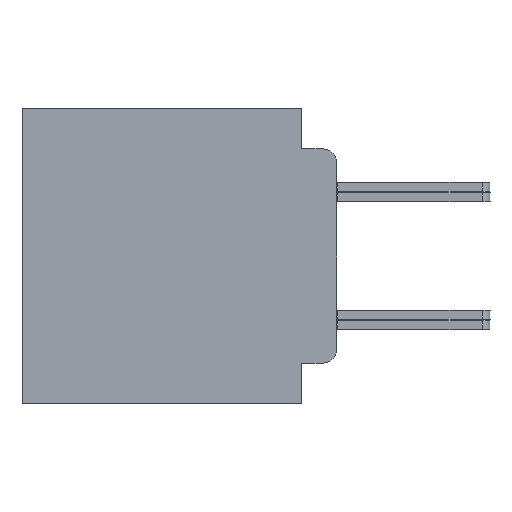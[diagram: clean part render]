
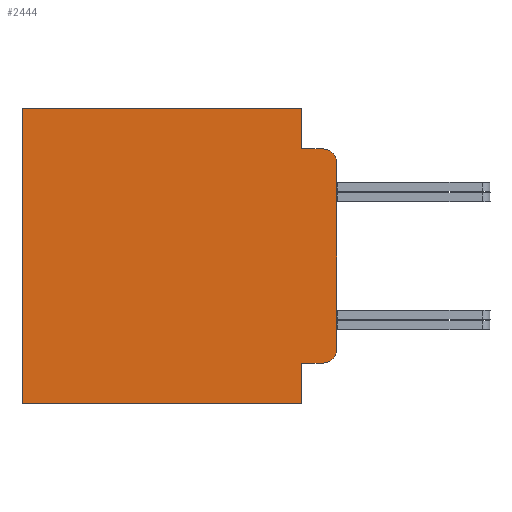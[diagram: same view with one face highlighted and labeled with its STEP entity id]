
A CAD part, left-side view. The second image highlights one B-rep face of the part: STEP entity #2444.
In plain terms, the highlighted planar face has unit normal (-1, 0, 0).
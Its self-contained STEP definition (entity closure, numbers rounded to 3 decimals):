
#29 = VERTEX_POINT ( 'NONE', #157 ) ;
#91 = EDGE_CURVE ( 'NONE', #19798, #8609, #27582, .T. ) ;
#157 = CARTESIAN_POINT ( 'NONE',  ( -67.462, 0., -3.467 ) ) ;
#174 = CARTESIAN_POINT ( 'NONE',  ( -67.462, 1.295, -3.975 ) ) ;
#429 = ORIENTED_EDGE ( 'NONE', *, *, #22593, .F. ) ;
#499 = VERTEX_POINT ( 'NONE', #3277 ) ;
#1486 = VERTEX_POINT ( 'NONE', #13337 ) ;
#2215 = CARTESIAN_POINT ( 'NONE',  ( -67.462, 0.508, 3.467 ) ) ;
#2444 = ADVANCED_FACE ( 'NONE', ( #26117 ), #5662, .F. ) ;
#3277 = CARTESIAN_POINT ( 'NONE',  ( -67.462, 0.508, -3.975 ) ) ;
#3463 = CARTESIAN_POINT ( 'NONE',  ( -67.462, 0., -5.486 ) ) ;
#3476 = CARTESIAN_POINT ( 'NONE',  ( -67.462, 1.295, 0. ) ) ;
#3770 = CARTESIAN_POINT ( 'NONE',  ( -67.462, 1.295, 0. ) ) ;
#4053 = DIRECTION ( 'NONE',  ( 0., 0., -1. ) ) ;
#4057 = LINE ( 'NONE', #3476, #26581 ) ;
#4779 = CARTESIAN_POINT ( 'NONE',  ( -67.462, 1.295, -5.486 ) ) ;
#5070 = LINE ( 'NONE', #24773, #21764 ) ;
#5470 = DIRECTION ( 'NONE',  ( 0., 0., -1. ) ) ;
#5475 = LINE ( 'NONE', #3463, #10943 ) ;
#5662 = PLANE ( 'NONE',  #19592 ) ;
#5704 = LINE ( 'NONE', #23634, #21716 ) ;
#5741 = VECTOR ( 'NONE', #18040, 1000. ) ;
#5996 = EDGE_CURVE ( 'NONE', #14584, #23016, #4057, .T. ) ;
#7024 = EDGE_CURVE ( 'NONE', #23016, #8609, #5070, .T. ) ;
#7458 = CARTESIAN_POINT ( 'NONE',  ( -67.462, 11.684, 5.486 ) ) ;
#8059 = CARTESIAN_POINT ( 'NONE',  ( -67.462, 0., -5.486 ) ) ;
#8399 = EDGE_CURVE ( 'NONE', #19581, #1486, #12910, .T. ) ;
#8609 = VERTEX_POINT ( 'NONE', #19529 ) ;
#8669 = ORIENTED_EDGE ( 'NONE', *, *, #8399, .F. ) ;
#8825 = VECTOR ( 'NONE', #16134, 1000. ) ;
#8961 = VERTEX_POINT ( 'NONE', #10941 ) ;
#9251 = ORIENTED_EDGE ( 'NONE', *, *, #16383, .T. ) ;
#9368 = CARTESIAN_POINT ( 'NONE',  ( -67.462, 11.684, -5.486 ) ) ;
#9481 = VERTEX_POINT ( 'NONE', #14904 ) ;
#9667 = VECTOR ( 'NONE', #16629, 1000. ) ;
#9810 = CARTESIAN_POINT ( 'NONE',  ( -67.462, 1.295, -3.975 ) ) ;
#10787 = ORIENTED_EDGE ( 'NONE', *, *, #26650, .T. ) ;
#10941 = CARTESIAN_POINT ( 'NONE',  ( -67.462, 1.295, 5.486 ) ) ;
#10943 = VECTOR ( 'NONE', #5470, 1000. ) ;
#12739 = LINE ( 'NONE', #9810, #19882 ) ;
#12910 = LINE ( 'NONE', #18489, #8825 ) ;
#13057 = CIRCLE ( 'NONE', #13110, 0.508 ) ;
#13110 = AXIS2_PLACEMENT_3D ( 'NONE', #21670, #28007, #4053 ) ;
#13337 = CARTESIAN_POINT ( 'NONE',  ( -67.462, 0.508, 3.975 ) ) ;
#14584 = VERTEX_POINT ( 'NONE', #174 ) ;
#14904 = CARTESIAN_POINT ( 'NONE',  ( -67.462, 0., 3.467 ) ) ;
#15452 = LINE ( 'NONE', #3770, #9667 ) ;
#15953 = ORIENTED_EDGE ( 'NONE', *, *, #22937, .T. ) ;
#16134 = DIRECTION ( 'NONE',  ( 0., -1., 0. ) ) ;
#16239 = EDGE_CURVE ( 'NONE', #8961, #19581, #15452, .T. ) ;
#16383 = EDGE_CURVE ( 'NONE', #499, #29, #13057, .T. ) ;
#16629 = DIRECTION ( 'NONE',  ( 0., 0., -1. ) ) ;
#17182 = DIRECTION ( 'NONE',  ( -1., 0., 0. ) ) ;
#17881 = ORIENTED_EDGE ( 'NONE', *, *, #5996, .F. ) ;
#17886 = ORIENTED_EDGE ( 'NONE', *, *, #91, .T. ) ;
#18040 = DIRECTION ( 'NONE',  ( 0., 0., -1. ) ) ;
#18489 = CARTESIAN_POINT ( 'NONE',  ( -67.462, 1.295, 3.975 ) ) ;
#18886 = DIRECTION ( 'NONE',  ( 1., 0., 0. ) ) ;
#18898 = ORIENTED_EDGE ( 'NONE', *, *, #16239, .F. ) ;
#19053 = AXIS2_PLACEMENT_3D ( 'NONE', #2215, #17182, #23769 ) ;
#19312 = ORIENTED_EDGE ( 'NONE', *, *, #20012, .T. ) ;
#19529 = CARTESIAN_POINT ( 'NONE',  ( -67.462, 11.684, -5.486 ) ) ;
#19581 = VERTEX_POINT ( 'NONE', #26354 ) ;
#19592 = AXIS2_PLACEMENT_3D ( 'NONE', #8059, #18886, #23289 ) ;
#19798 = VERTEX_POINT ( 'NONE', #7458 ) ;
#19882 = VECTOR ( 'NONE', #25231, 1000. ) ;
#20012 = EDGE_CURVE ( 'NONE', #8961, #19798, #5704, .T. ) ;
#20458 = DIRECTION ( 'NONE',  ( 0., 1., 0. ) ) ;
#21670 = CARTESIAN_POINT ( 'NONE',  ( -67.462, 0.508, -3.467 ) ) ;
#21716 = VECTOR ( 'NONE', #28156, 1000. ) ;
#21764 = VECTOR ( 'NONE', #20458, 1000. ) ;
#22513 = ORIENTED_EDGE ( 'NONE', *, *, #7024, .F. ) ;
#22593 = EDGE_CURVE ( 'NONE', #9481, #29, #5475, .T. ) ;
#22937 = EDGE_CURVE ( 'NONE', #9481, #1486, #25228, .T. ) ;
#23016 = VERTEX_POINT ( 'NONE', #4779 ) ;
#23289 = DIRECTION ( 'NONE',  ( 0., 0., -1. ) ) ;
#23634 = CARTESIAN_POINT ( 'NONE',  ( -67.462, 0., 5.486 ) ) ;
#23769 = DIRECTION ( 'NONE',  ( 0., 0., -1. ) ) ;
#24773 = CARTESIAN_POINT ( 'NONE',  ( -67.462, 0., -5.486 ) ) ;
#25228 = CIRCLE ( 'NONE', #19053, 0.508 ) ;
#25231 = DIRECTION ( 'NONE',  ( 0., -1., 0. ) ) ;
#25414 = DIRECTION ( 'NONE',  ( 0., 0., -1. ) ) ;
#26117 = FACE_OUTER_BOUND ( 'NONE', #27833, .T. ) ;
#26354 = CARTESIAN_POINT ( 'NONE',  ( -67.462, 1.295, 3.975 ) ) ;
#26581 = VECTOR ( 'NONE', #25414, 1000. ) ;
#26650 = EDGE_CURVE ( 'NONE', #14584, #499, #12739, .T. ) ;
#27582 = LINE ( 'NONE', #9368, #5741 ) ;
#27833 = EDGE_LOOP ( 'NONE', ( #10787, #9251, #429, #15953, #8669, #18898, #19312, #17886, #22513, #17881 ) ) ;
#28007 = DIRECTION ( 'NONE',  ( -1., 0., 0. ) ) ;
#28156 = DIRECTION ( 'NONE',  ( 0., 1., 0. ) ) ;
